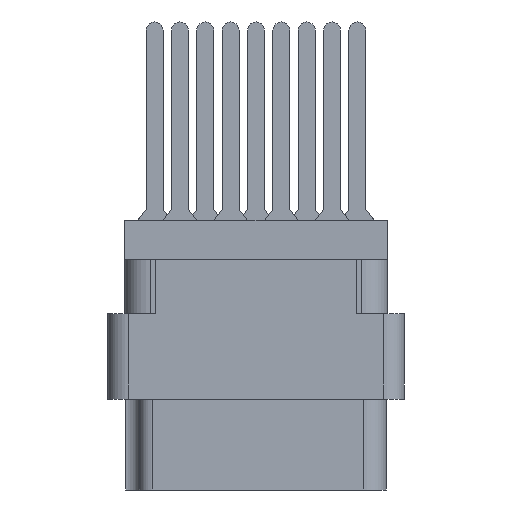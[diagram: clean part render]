
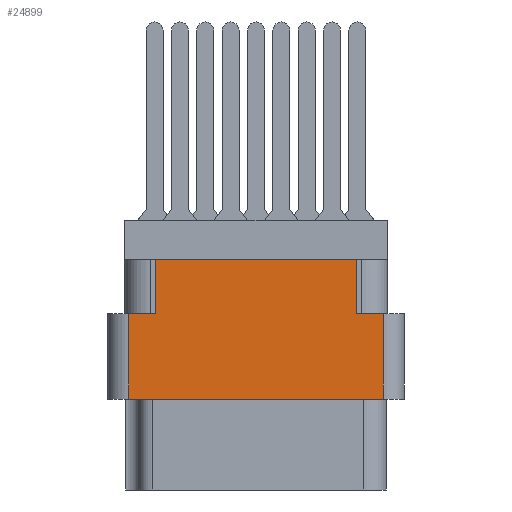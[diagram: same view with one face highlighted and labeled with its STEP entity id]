
A CAD part, left-side view. The second image highlights one B-rep face of the part: STEP entity #24899.
In plain terms, the highlighted planar face has unit normal (-1, 0, 0).
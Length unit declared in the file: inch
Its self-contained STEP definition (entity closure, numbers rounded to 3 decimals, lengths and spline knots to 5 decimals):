
#1065 = EDGE_LOOP ( 'NONE', ( #9236, #19428, #24997, #4374, #7336, #23461, #13579, #18185 ) ) ;
#1498 = LINE ( 'NONE', #32737, #29228 ) ;
#1507 = CARTESIAN_POINT ( 'NONE',  ( -1., 0.296, -0.117 ) ) ;
#3074 = LINE ( 'NONE', #16484, #17747 ) ;
#3384 = VERTEX_POINT ( 'NONE', #34334 ) ;
#3629 = EDGE_CURVE ( 'NONE', #22162, #28677, #3074, .T. ) ;
#3746 = CARTESIAN_POINT ( 'NONE',  ( -1., 0., -0.277 ) ) ;
#3876 = EDGE_CURVE ( 'NONE', #25652, #30148, #5129, .T. ) ;
#4004 = CARTESIAN_POINT ( 'NONE',  ( -1., -0.376, -0.277 ) ) ;
#4374 = ORIENTED_EDGE ( 'NONE', *, *, #3629, .T. ) ;
#4718 = PLANE ( 'NONE',  #33460 ) ;
#5129 = LINE ( 'NONE', #34417, #17709 ) ;
#5292 = EDGE_CURVE ( 'NONE', #23672, #22272, #14278, .T. ) ;
#6343 = EDGE_CURVE ( 'NONE', #22162, #30148, #33135, .T. ) ;
#7336 = ORIENTED_EDGE ( 'NONE', *, *, #17575, .F. ) ;
#7583 = CARTESIAN_POINT ( 'NONE',  ( -1., 0., -0.529 ) ) ;
#8272 = DIRECTION ( 'NONE',  ( 0., 0., 1. ) ) ;
#9236 = ORIENTED_EDGE ( 'NONE', *, *, #27430, .F. ) ;
#9265 = VECTOR ( 'NONE', #34220, 39.37008 ) ;
#9769 = EDGE_CURVE ( 'NONE', #22272, #34589, #31229, .T. ) ;
#9891 = CARTESIAN_POINT ( 'NONE',  ( -1., -0.438, -0.798 ) ) ;
#10234 = DIRECTION ( 'NONE',  ( -1., 0., 0. ) ) ;
#11460 = VECTOR ( 'NONE', #30446, 39.37008 ) ;
#11575 = CARTESIAN_POINT ( 'NONE',  ( -1., -0.376, -0.529 ) ) ;
#12940 = CARTESIAN_POINT ( 'NONE',  ( -1., -0.296, -0.277 ) ) ;
#13352 = CARTESIAN_POINT ( 'NONE',  ( -1., 0.296, -0.277 ) ) ;
#13579 = ORIENTED_EDGE ( 'NONE', *, *, #9769, .F. ) ;
#13980 = CARTESIAN_POINT ( 'NONE',  ( -1., -0.296, -0.117 ) ) ;
#14278 = LINE ( 'NONE', #30025, #14674 ) ;
#14674 = VECTOR ( 'NONE', #16730, 39.37008 ) ;
#16484 = CARTESIAN_POINT ( 'NONE',  ( -1., -0.376, -0.798 ) ) ;
#16730 = DIRECTION ( 'NONE',  ( 0., 0., 1. ) ) ;
#17575 = EDGE_CURVE ( 'NONE', #3384, #28677, #1498, .T. ) ;
#17709 = VECTOR ( 'NONE', #26104, 39.37008 ) ;
#17747 = VECTOR ( 'NONE', #8272, 39.37008 ) ;
#18185 = ORIENTED_EDGE ( 'NONE', *, *, #5292, .F. ) ;
#19428 = ORIENTED_EDGE ( 'NONE', *, *, #3876, .T. ) ;
#19458 = DIRECTION ( 'NONE',  ( 0., -1., 0. ) ) ;
#20670 = DIRECTION ( 'NONE',  ( 0., 1., 0. ) ) ;
#21616 = CARTESIAN_POINT ( 'NONE',  ( -1., 0.376, -0.277 ) ) ;
#21827 = VECTOR ( 'NONE', #20670, 39.37008 ) ;
#22162 = VERTEX_POINT ( 'NONE', #11575 ) ;
#22272 = VERTEX_POINT ( 'NONE', #1507 ) ;
#22756 = DIRECTION ( 'NONE',  ( 0., -1., 0. ) ) ;
#22919 = CARTESIAN_POINT ( 'NONE',  ( -1., 0.438, -0.117 ) ) ;
#23461 = ORIENTED_EDGE ( 'NONE', *, *, #32633, .T. ) ;
#23531 = DIRECTION ( 'NONE',  ( 0., 0., 1. ) ) ;
#23672 = VERTEX_POINT ( 'NONE', #13352 ) ;
#24894 = CARTESIAN_POINT ( 'NONE',  ( -1., 0.376, -0.529 ) ) ;
#24899 = ADVANCED_FACE ( 'NONE', ( #25099 ), #4718, .T. ) ;
#24997 = ORIENTED_EDGE ( 'NONE', *, *, #6343, .F. ) ;
#25099 = FACE_OUTER_BOUND ( 'NONE', #1065, .T. ) ;
#25652 = VERTEX_POINT ( 'NONE', #21616 ) ;
#26104 = DIRECTION ( 'NONE',  ( 0., 0., -1. ) ) ;
#26733 = VECTOR ( 'NONE', #22756, 39.37008 ) ;
#27430 = EDGE_CURVE ( 'NONE', #25652, #23672, #34690, .T. ) ;
#28677 = VERTEX_POINT ( 'NONE', #4004 ) ;
#29228 = VECTOR ( 'NONE', #19458, 39.37008 ) ;
#29884 = LINE ( 'NONE', #12940, #9265 ) ;
#30025 = CARTESIAN_POINT ( 'NONE',  ( -1., 0.296, -0.277 ) ) ;
#30148 = VERTEX_POINT ( 'NONE', #24894 ) ;
#30446 = DIRECTION ( 'NONE',  ( 0., -1., 0. ) ) ;
#31229 = LINE ( 'NONE', #22919, #11460 ) ;
#32633 = EDGE_CURVE ( 'NONE', #3384, #34589, #29884, .T. ) ;
#32737 = CARTESIAN_POINT ( 'NONE',  ( -1., 0., -0.277 ) ) ;
#33135 = LINE ( 'NONE', #7583, #21827 ) ;
#33460 = AXIS2_PLACEMENT_3D ( 'NONE', #9891, #10234, #23531 ) ;
#34220 = DIRECTION ( 'NONE',  ( 0., 0., 1. ) ) ;
#34334 = CARTESIAN_POINT ( 'NONE',  ( -1., -0.296, -0.277 ) ) ;
#34417 = CARTESIAN_POINT ( 'NONE',  ( -1., 0.376, -0.798 ) ) ;
#34589 = VERTEX_POINT ( 'NONE', #13980 ) ;
#34690 = LINE ( 'NONE', #3746, #26733 ) ;
